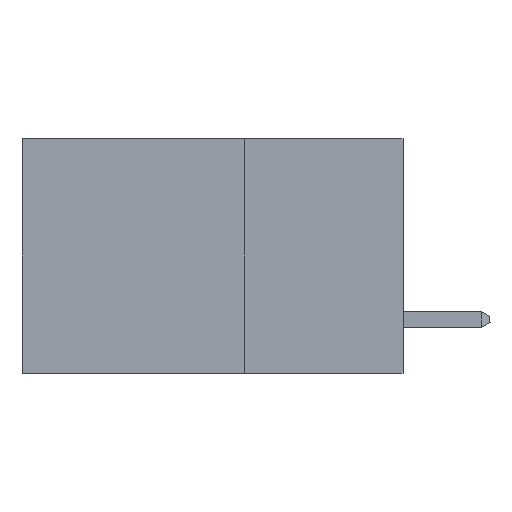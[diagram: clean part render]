
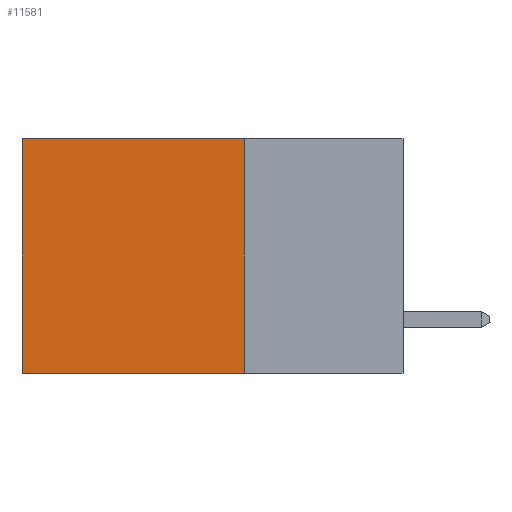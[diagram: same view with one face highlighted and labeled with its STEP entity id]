
A CAD part, left-side view. The second image highlights one B-rep face of the part: STEP entity #11581.
In plain terms, the highlighted planar face has unit normal (-1, 0, 0).
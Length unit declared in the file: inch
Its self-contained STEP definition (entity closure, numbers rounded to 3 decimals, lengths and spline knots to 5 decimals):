
#3966 = CARTESIAN_POINT ( 'NONE',  ( 0.2875, 0.25, -0.37 ) ) ;
#4696 = LINE ( 'NONE', #3966, #18840 ) ;
#7708 = FACE_OUTER_BOUND ( 'NONE', #40647, .T. ) ;
#8080 = VECTOR ( 'NONE', #27901, 39.37008 ) ;
#8137 = CARTESIAN_POINT ( 'NONE',  ( 0.2875, 0.25, 0. ) ) ;
#8375 = CARTESIAN_POINT ( 'NONE',  ( 0.2875, 0.6, 0. ) ) ;
#8825 = CARTESIAN_POINT ( 'NONE',  ( 0.2875, 0.6, 0. ) ) ;
#9343 = ORIENTED_EDGE ( 'NONE', *, *, #37372, .F. ) ;
#9816 = EDGE_CURVE ( 'NONE', #22767, #31058, #33250, .T. ) ;
#10321 = CARTESIAN_POINT ( 'NONE',  ( 0.2875, 0.25, 0. ) ) ;
#10612 = DIRECTION ( 'NONE',  ( 1., 0., 0. ) ) ;
#10941 = VECTOR ( 'NONE', #14978, 39.37008 ) ;
#11581 = ADVANCED_FACE ( 'NONE', ( #7708 ), #24484, .F. ) ;
#11800 = DIRECTION ( 'NONE',  ( 0., 1., 0. ) ) ;
#14890 = LINE ( 'NONE', #8137, #10941 ) ;
#14978 = DIRECTION ( 'NONE',  ( 0., 1., 0. ) ) ;
#16406 = CARTESIAN_POINT ( 'NONE',  ( 0.2875, 0.25, 0. ) ) ;
#17889 = AXIS2_PLACEMENT_3D ( 'NONE', #10321, #10612, #25538 ) ;
#18840 = VECTOR ( 'NONE', #11800, 39.37008 ) ;
#21263 = VERTEX_POINT ( 'NONE', #16406 ) ;
#21282 = ORIENTED_EDGE ( 'NONE', *, *, #31206, .T. ) ;
#22148 = EDGE_CURVE ( 'NONE', #21263, #24125, #36579, .T. ) ;
#22767 = VERTEX_POINT ( 'NONE', #8825 ) ;
#23142 = DIRECTION ( 'NONE',  ( 0., 0., -1. ) ) ;
#24125 = VERTEX_POINT ( 'NONE', #38095 ) ;
#24484 = PLANE ( 'NONE',  #17889 ) ;
#25538 = DIRECTION ( 'NONE',  ( 0., 0., -1. ) ) ;
#26628 = ORIENTED_EDGE ( 'NONE', *, *, #9816, .T. ) ;
#27901 = DIRECTION ( 'NONE',  ( 0., 0., -1. ) ) ;
#30395 = CARTESIAN_POINT ( 'NONE',  ( 0.2875, 0.25, 0. ) ) ;
#31058 = VERTEX_POINT ( 'NONE', #44734 ) ;
#31206 = EDGE_CURVE ( 'NONE', #21263, #22767, #14890, .T. ) ;
#33250 = LINE ( 'NONE', #8375, #40659 ) ;
#36579 = LINE ( 'NONE', #30395, #8080 ) ;
#37372 = EDGE_CURVE ( 'NONE', #24125, #31058, #4696, .T. ) ;
#38095 = CARTESIAN_POINT ( 'NONE',  ( 0.2875, 0.25, -0.37 ) ) ;
#40187 = ORIENTED_EDGE ( 'NONE', *, *, #22148, .F. ) ;
#40647 = EDGE_LOOP ( 'NONE', ( #26628, #9343, #40187, #21282 ) ) ;
#40659 = VECTOR ( 'NONE', #23142, 39.37008 ) ;
#44734 = CARTESIAN_POINT ( 'NONE',  ( 0.2875, 0.6, -0.37 ) ) ;
